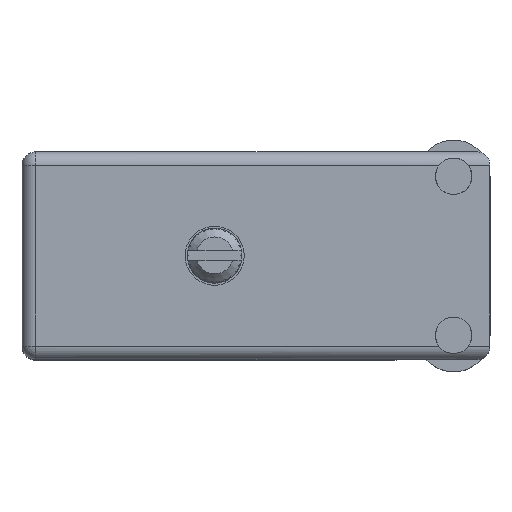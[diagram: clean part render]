
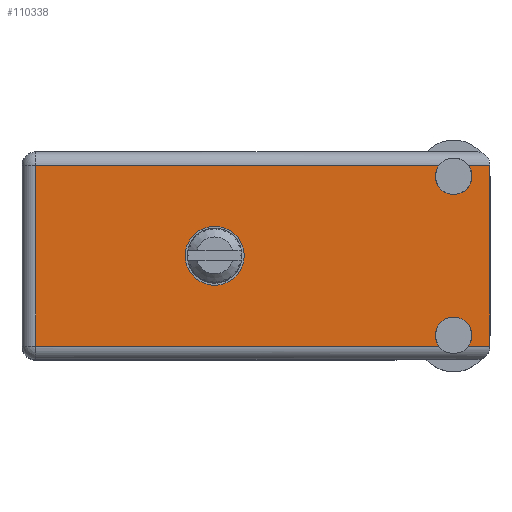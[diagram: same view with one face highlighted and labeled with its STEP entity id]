
A CAD part, top view. The second image highlights one B-rep face of the part: STEP entity #110338.
In plain terms, the highlighted face is planar.
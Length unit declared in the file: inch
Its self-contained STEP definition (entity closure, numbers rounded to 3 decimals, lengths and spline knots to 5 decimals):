
#837 = VECTOR ( 'NONE', #83554, 39.37008 ) ;
#1623 = VERTEX_POINT ( 'NONE', #54655 ) ;
#4106 = VERTEX_POINT ( 'NONE', #29487 ) ;
#8864 = VERTEX_POINT ( 'NONE', #35200 ) ;
#11790 = CARTESIAN_POINT ( 'NONE',  ( 0.6625, 0.906, -0.3575 ) ) ;
#13075 = ORIENTED_EDGE ( 'NONE', *, *, #165739, .T. ) ;
#14074 = DIRECTION ( 'NONE',  ( 0., 1., 0. ) ) ;
#14561 = CARTESIAN_POINT ( 'NONE',  ( 1.609, 0.906, -0.047 ) ) ;
#16164 = DIRECTION ( 'NONE',  ( 0., 0., 1. ) ) ;
#19527 = CARTESIAN_POINT ( 'NONE',  ( 1.609, 0.906, -0.047 ) ) ;
#20282 = CIRCLE ( 'NONE', #68978, 0.1015 ) ;
#21740 = EDGE_CURVE ( 'NONE', #26325, #117189, #115683, .T. ) ;
#23621 = EDGE_CURVE ( 'NONE', #129757, #8864, #144450, .T. ) ;
#26325 = VERTEX_POINT ( 'NONE', #158242 ) ;
#27924 = DIRECTION ( 'NONE',  ( 0., 0., 1. ) ) ;
#29487 = CARTESIAN_POINT ( 'NONE',  ( 1.609, 0.906, -0.047 ) ) ;
#31267 = CARTESIAN_POINT ( 'NONE',  ( 0., 0.906, -0.715 ) ) ;
#31894 = ORIENTED_EDGE ( 'NONE', *, *, #23621, .T. ) ;
#32288 = LINE ( 'NONE', #173745, #119758 ) ;
#32668 = DIRECTION ( 'NONE',  ( -1., 0., 0. ) ) ;
#32915 = VERTEX_POINT ( 'NONE', #56522 ) ;
#33806 = VECTOR ( 'NONE', #32668, 39.37008 ) ;
#34387 = ORIENTED_EDGE ( 'NONE', *, *, #84649, .F. ) ;
#35200 = CARTESIAN_POINT ( 'NONE',  ( 0.047, 0.906, -0.047 ) ) ;
#37440 = CARTESIAN_POINT ( 'NONE',  ( 1.484, 0.906, -0.631 ) ) ;
#38657 = DIRECTION ( 'NONE',  ( 0., 0., 1. ) ) ;
#41541 = EDGE_LOOP ( 'NONE', ( #69263, #61985 ) ) ;
#45544 = CARTESIAN_POINT ( 'NONE',  ( 0.6625, 0.906, -0.459 ) ) ;
#45972 = ORIENTED_EDGE ( 'NONE', *, *, #113046, .T. ) ;
#47128 = CARTESIAN_POINT ( 'NONE',  ( 1.53437, 0.906, -0.047 ) ) ;
#47600 = EDGE_LOOP ( 'NONE', ( #64354, #69135, #113375, #113434, #34387, #45972, #76744, #109323, #13075, #31894 ) ) ;
#47826 = AXIS2_PLACEMENT_3D ( 'NONE', #37440, #66263, #38657 ) ;
#54655 = CARTESIAN_POINT ( 'NONE',  ( 1.609, 0.906, -0.668 ) ) ;
#56522 = CARTESIAN_POINT ( 'NONE',  ( 0.6625, 0.906, -0.256 ) ) ;
#56909 = VECTOR ( 'NONE', #27924, 39.37008 ) ;
#58721 = CARTESIAN_POINT ( 'NONE',  ( 1.484, 0.906, -0.631 ) ) ;
#59044 = LINE ( 'NONE', #14561, #837 ) ;
#60880 = FACE_BOUND ( 'NONE', #41541, .T. ) ;
#61985 = ORIENTED_EDGE ( 'NONE', *, *, #177127, .F. ) ;
#64354 = ORIENTED_EDGE ( 'NONE', *, *, #97905, .T. ) ;
#64374 = LINE ( 'NONE', #19527, #107055 ) ;
#66104 = CIRCLE ( 'NONE', #75555, 0.0625 ) ;
#66263 = DIRECTION ( 'NONE',  ( 0., 1., 0. ) ) ;
#68978 = AXIS2_PLACEMENT_3D ( 'NONE', #11790, #98362, #182419 ) ;
#69135 = ORIENTED_EDGE ( 'NONE', *, *, #130906, .F. ) ;
#69263 = ORIENTED_EDGE ( 'NONE', *, *, #113242, .F. ) ;
#74481 = DIRECTION ( 'NONE',  ( 0., 1., 0. ) ) ;
#75555 = AXIS2_PLACEMENT_3D ( 'NONE', #178299, #150093, #108021 ) ;
#76744 = ORIENTED_EDGE ( 'NONE', *, *, #108290, .F. ) ;
#77089 = CARTESIAN_POINT ( 'NONE',  ( 0., 0.906, -0.668 ) ) ;
#78951 = VERTEX_POINT ( 'NONE', #45544 ) ;
#81591 = CARTESIAN_POINT ( 'NONE',  ( 0.6625, 0.906, -0.3575 ) ) ;
#83554 = DIRECTION ( 'NONE',  ( 1., 0., 0. ) ) ;
#83985 = CARTESIAN_POINT ( 'NONE',  ( 1.53437, 0.906, -0.668 ) ) ;
#84649 = EDGE_CURVE ( 'NONE', #1623, #4106, #174412, .T. ) ;
#85842 = AXIS2_PLACEMENT_3D ( 'NONE', #81591, #111701, #126796 ) ;
#90931 = VERTEX_POINT ( 'NONE', #101805 ) ;
#97723 = CARTESIAN_POINT ( 'NONE',  ( 1.609, 0.906, 0. ) ) ;
#97905 = EDGE_CURVE ( 'NONE', #8864, #90931, #64374, .T. ) ;
#98362 = DIRECTION ( 'NONE',  ( 0., 1., 0. ) ) ;
#101805 = CARTESIAN_POINT ( 'NONE',  ( 1.43363, 0.906, -0.047 ) ) ;
#103594 = DIRECTION ( 'NONE',  ( 1., 0., 0. ) ) ;
#105818 = AXIS2_PLACEMENT_3D ( 'NONE', #183352, #14074, #183822 ) ;
#107055 = VECTOR ( 'NONE', #103594, 39.37008 ) ;
#108021 = DIRECTION ( 'NONE',  ( 0., 0., 1. ) ) ;
#108290 = EDGE_CURVE ( 'NONE', #117189, #131924, #124131, .T. ) ;
#109323 = ORIENTED_EDGE ( 'NONE', *, *, #21740, .F. ) ;
#109430 = AXIS2_PLACEMENT_3D ( 'NONE', #58721, #159158, #16164 ) ;
#110338 = ADVANCED_FACE ( 'NONE', ( #60880, #135322 ), #116006, .T. ) ;
#111701 = DIRECTION ( 'NONE',  ( 0., 1., 0. ) ) ;
#113046 = EDGE_CURVE ( 'NONE', #1623, #131924, #125979, .T. ) ;
#113242 = EDGE_CURVE ( 'NONE', #32915, #78951, #20282, .T. ) ;
#113375 = ORIENTED_EDGE ( 'NONE', *, *, #139465, .F. ) ;
#113434 = ORIENTED_EDGE ( 'NONE', *, *, #132514, .T. ) ;
#113824 = CARTESIAN_POINT ( 'NONE',  ( 0.047, 0.906, -0.668 ) ) ;
#115301 = CARTESIAN_POINT ( 'NONE',  ( 1.484, 0.906, -0.1465 ) ) ;
#115683 = CIRCLE ( 'NONE', #109430, 0.0625 ) ;
#116006 = PLANE ( 'NONE',  #166026 ) ;
#117189 = VERTEX_POINT ( 'NONE', #175663 ) ;
#119758 = VECTOR ( 'NONE', #174973, 39.37008 ) ;
#124131 = CIRCLE ( 'NONE', #47826, 0.0625 ) ;
#125979 = LINE ( 'NONE', #77089, #33806 ) ;
#126662 = DIRECTION ( 'NONE',  ( 0., 0., 1. ) ) ;
#126796 = DIRECTION ( 'NONE',  ( 0., 0., 1. ) ) ;
#129538 = CARTESIAN_POINT ( 'NONE',  ( 0.047, 0.906, -0.715 ) ) ;
#129757 = VERTEX_POINT ( 'NONE', #113824 ) ;
#130906 = EDGE_CURVE ( 'NONE', #160006, #90931, #66104, .T. ) ;
#131924 = VERTEX_POINT ( 'NONE', #83985 ) ;
#132514 = EDGE_CURVE ( 'NONE', #159531, #4106, #59044, .T. ) ;
#134058 = CIRCLE ( 'NONE', #85842, 0.1015 ) ;
#135322 = FACE_OUTER_BOUND ( 'NONE', #47600, .T. ) ;
#136245 = VECTOR ( 'NONE', #126662, 39.37008 ) ;
#139465 = EDGE_CURVE ( 'NONE', #159531, #160006, #141468, .T. ) ;
#141468 = CIRCLE ( 'NONE', #105818, 0.0625 ) ;
#144450 = LINE ( 'NONE', #129538, #56909 ) ;
#150093 = DIRECTION ( 'NONE',  ( 0., 1., 0. ) ) ;
#158242 = CARTESIAN_POINT ( 'NONE',  ( 1.43363, 0.906, -0.668 ) ) ;
#159158 = DIRECTION ( 'NONE',  ( 0., 1., 0. ) ) ;
#159531 = VERTEX_POINT ( 'NONE', #47128 ) ;
#160006 = VERTEX_POINT ( 'NONE', #115301 ) ;
#165739 = EDGE_CURVE ( 'NONE', #26325, #129757, #32288, .T. ) ;
#166026 = AXIS2_PLACEMENT_3D ( 'NONE', #31267, #74481, #174914 ) ;
#173745 = CARTESIAN_POINT ( 'NONE',  ( 0., 0.906, -0.668 ) ) ;
#174412 = LINE ( 'NONE', #97723, #136245 ) ;
#174914 = DIRECTION ( 'NONE',  ( 0., 0., 1. ) ) ;
#174973 = DIRECTION ( 'NONE',  ( -1., 0., 0. ) ) ;
#175663 = CARTESIAN_POINT ( 'NONE',  ( 1.484, 0.906, -0.5685 ) ) ;
#177127 = EDGE_CURVE ( 'NONE', #78951, #32915, #134058, .T. ) ;
#178299 = CARTESIAN_POINT ( 'NONE',  ( 1.484, 0.906, -0.084 ) ) ;
#182419 = DIRECTION ( 'NONE',  ( 0., 0., 1. ) ) ;
#183352 = CARTESIAN_POINT ( 'NONE',  ( 1.484, 0.906, -0.084 ) ) ;
#183822 = DIRECTION ( 'NONE',  ( 0., 0., 1. ) ) ;
